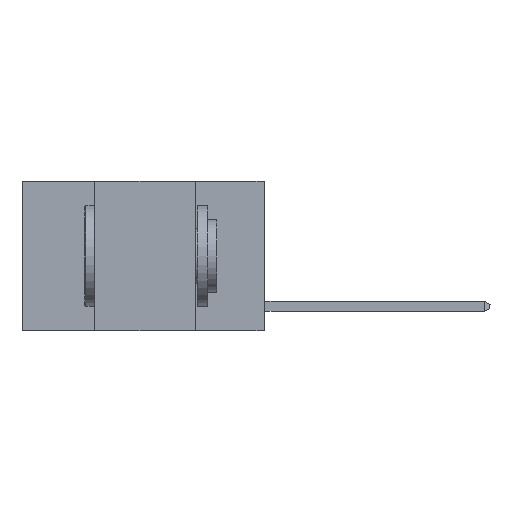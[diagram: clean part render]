
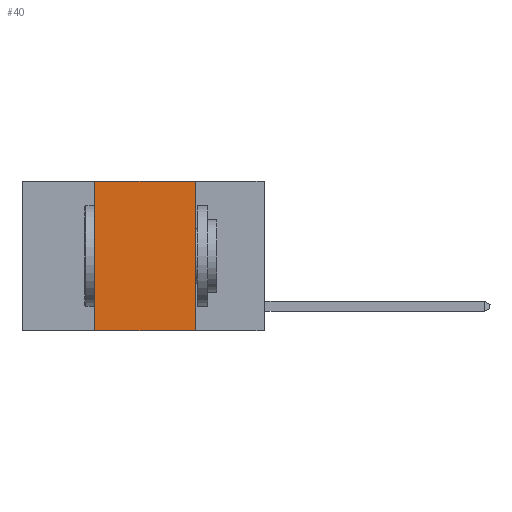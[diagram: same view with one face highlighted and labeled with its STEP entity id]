
A CAD part, left-side view. The second image highlights one B-rep face of the part: STEP entity #40.
In plain terms, the highlighted planar face has unit normal (-1, 0, 0).
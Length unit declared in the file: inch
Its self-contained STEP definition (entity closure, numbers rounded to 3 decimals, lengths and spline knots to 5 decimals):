
#40 = ADVANCED_FACE ( 'NONE', ( #1677 ), #8229, .F. ) ;
#136 = CARTESIAN_POINT ( 'NONE',  ( 0., 0.42, 0. ) ) ;
#380 = CARTESIAN_POINT ( 'NONE',  ( 0., 0.6, -0.37 ) ) ;
#680 = CARTESIAN_POINT ( 'NONE',  ( 0., 0.6, 0. ) ) ;
#1545 = VECTOR ( 'NONE', #9575, 39.37008 ) ;
#1677 = FACE_OUTER_BOUND ( 'NONE', #8202, .T. ) ;
#1852 = ORIENTED_EDGE ( 'NONE', *, *, #8104, .F. ) ;
#1893 = CARTESIAN_POINT ( 'NONE',  ( 0., 0.17, 0. ) ) ;
#1941 = LINE ( 'NONE', #380, #1545 ) ;
#2294 = DIRECTION ( 'NONE',  ( 1., 0., 0. ) ) ;
#2566 = LINE ( 'NONE', #1893, #8972 ) ;
#2937 = CARTESIAN_POINT ( 'NONE',  ( 0., 0.17, 0. ) ) ;
#4291 = DIRECTION ( 'NONE',  ( 0., 0., -1. ) ) ;
#4308 = VECTOR ( 'NONE', #6999, 39.37008 ) ;
#4478 = ORIENTED_EDGE ( 'NONE', *, *, #9072, .T. ) ;
#4699 = EDGE_CURVE ( 'NONE', #4814, #8611, #6272, .T. ) ;
#4814 = VERTEX_POINT ( 'NONE', #136 ) ;
#5728 = EDGE_CURVE ( 'NONE', #8611, #6895, #2566, .T. ) ;
#6272 = LINE ( 'NONE', #7823, #4308 ) ;
#6347 = DIRECTION ( 'NONE',  ( 0., 0., 1. ) ) ;
#6724 = CARTESIAN_POINT ( 'NONE',  ( 0., 0.17, -0.37 ) ) ;
#6858 = VECTOR ( 'NONE', #6347, 39.37008 ) ;
#6895 = VERTEX_POINT ( 'NONE', #6724 ) ;
#6999 = DIRECTION ( 'NONE',  ( 0., -1., 0. ) ) ;
#7255 = LINE ( 'NONE', #8833, #6858 ) ;
#7425 = CARTESIAN_POINT ( 'NONE',  ( 0., 0.42, -0.37 ) ) ;
#7823 = CARTESIAN_POINT ( 'NONE',  ( 0., 0.6, 0. ) ) ;
#7869 = AXIS2_PLACEMENT_3D ( 'NONE', #680, #2294, #10617 ) ;
#8104 = EDGE_CURVE ( 'NONE', #10643, #4814, #7255, .T. ) ;
#8202 = EDGE_LOOP ( 'NONE', ( #9029, #8880, #1852, #4478 ) ) ;
#8229 = PLANE ( 'NONE',  #7869 ) ;
#8611 = VERTEX_POINT ( 'NONE', #2937 ) ;
#8833 = CARTESIAN_POINT ( 'NONE',  ( 0., 0.42, 0. ) ) ;
#8880 = ORIENTED_EDGE ( 'NONE', *, *, #4699, .F. ) ;
#8972 = VECTOR ( 'NONE', #4291, 39.37008 ) ;
#9029 = ORIENTED_EDGE ( 'NONE', *, *, #5728, .F. ) ;
#9072 = EDGE_CURVE ( 'NONE', #10643, #6895, #1941, .T. ) ;
#9575 = DIRECTION ( 'NONE',  ( 0., -1., 0. ) ) ;
#10617 = DIRECTION ( 'NONE',  ( 0., 0., -1. ) ) ;
#10643 = VERTEX_POINT ( 'NONE', #7425 ) ;
